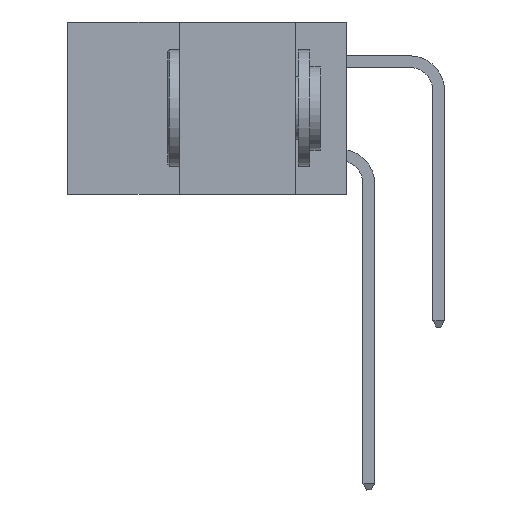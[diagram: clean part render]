
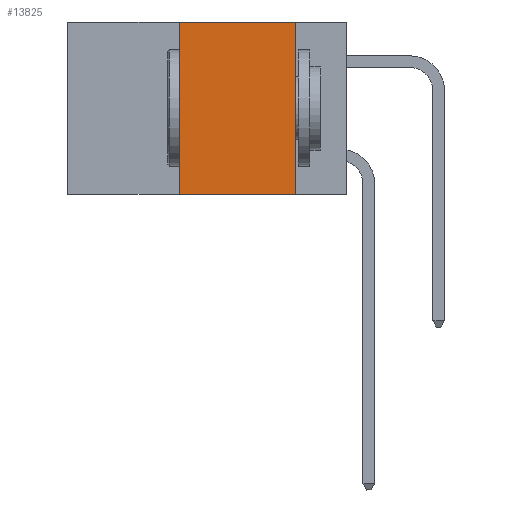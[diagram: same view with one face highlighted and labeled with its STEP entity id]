
A CAD part, left-side view. The second image highlights one B-rep face of the part: STEP entity #13825.
In plain terms, the highlighted planar face has unit normal (-1, 0, 0).
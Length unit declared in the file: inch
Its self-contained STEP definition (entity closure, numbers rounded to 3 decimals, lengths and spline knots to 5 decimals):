
#521 = VECTOR ( 'NONE', #5944, 39.37008 ) ;
#1045 = CARTESIAN_POINT ( 'NONE',  ( 0., 0.36, 0. ) ) ;
#1995 = EDGE_CURVE ( 'NONE', #41050, #14341, #8849, .T. ) ;
#2051 = CARTESIAN_POINT ( 'NONE',  ( 0., 0.11, -0.37 ) ) ;
#2618 = CARTESIAN_POINT ( 'NONE',  ( 0., 0.6, -0.37 ) ) ;
#5733 = AXIS2_PLACEMENT_3D ( 'NONE', #9460, #19640, #33108 ) ;
#5944 = DIRECTION ( 'NONE',  ( 0., -1., 0. ) ) ;
#8849 = LINE ( 'NONE', #2618, #521 ) ;
#9460 = CARTESIAN_POINT ( 'NONE',  ( 0., 0.6, 0. ) ) ;
#10995 = EDGE_CURVE ( 'NONE', #20902, #42044, #36940, .T. ) ;
#13240 = PLANE ( 'NONE',  #5733 ) ;
#13600 = LINE ( 'NONE', #1045, #28740 ) ;
#13825 = ADVANCED_FACE ( 'NONE', ( #15159 ), #13240, .F. ) ;
#14341 = VERTEX_POINT ( 'NONE', #2051 ) ;
#14411 = DIRECTION ( 'NONE',  ( 0., 0., 1. ) ) ;
#14940 = VECTOR ( 'NONE', #39804, 39.37008 ) ;
#14994 = ORIENTED_EDGE ( 'NONE', *, *, #40421, .F. ) ;
#15159 = FACE_OUTER_BOUND ( 'NONE', #24871, .T. ) ;
#17539 = ORIENTED_EDGE ( 'NONE', *, *, #42291, .F. ) ;
#19640 = DIRECTION ( 'NONE',  ( 1., 0., 0. ) ) ;
#20674 = CARTESIAN_POINT ( 'NONE',  ( 0., 0.11, 0. ) ) ;
#20902 = VERTEX_POINT ( 'NONE', #39562 ) ;
#22892 = VECTOR ( 'NONE', #37954, 39.37008 ) ;
#23579 = ORIENTED_EDGE ( 'NONE', *, *, #10995, .F. ) ;
#24871 = EDGE_LOOP ( 'NONE', ( #14994, #23579, #17539, #41478 ) ) ;
#28740 = VECTOR ( 'NONE', #14411, 39.37008 ) ;
#29167 = LINE ( 'NONE', #20674, #22892 ) ;
#33108 = DIRECTION ( 'NONE',  ( 0., 0., -1. ) ) ;
#35795 = CARTESIAN_POINT ( 'NONE',  ( 0., 0.11, 0. ) ) ;
#36744 = CARTESIAN_POINT ( 'NONE',  ( 0., 0.6, 0. ) ) ;
#36940 = LINE ( 'NONE', #36744, #14940 ) ;
#37954 = DIRECTION ( 'NONE',  ( 0., 0., -1. ) ) ;
#39562 = CARTESIAN_POINT ( 'NONE',  ( 0., 0.36, 0. ) ) ;
#39804 = DIRECTION ( 'NONE',  ( 0., -1., 0. ) ) ;
#40421 = EDGE_CURVE ( 'NONE', #42044, #14341, #29167, .T. ) ;
#41050 = VERTEX_POINT ( 'NONE', #41549 ) ;
#41478 = ORIENTED_EDGE ( 'NONE', *, *, #1995, .T. ) ;
#41549 = CARTESIAN_POINT ( 'NONE',  ( 0., 0.36, -0.37 ) ) ;
#42044 = VERTEX_POINT ( 'NONE', #35795 ) ;
#42291 = EDGE_CURVE ( 'NONE', #41050, #20902, #13600, .T. ) ;
